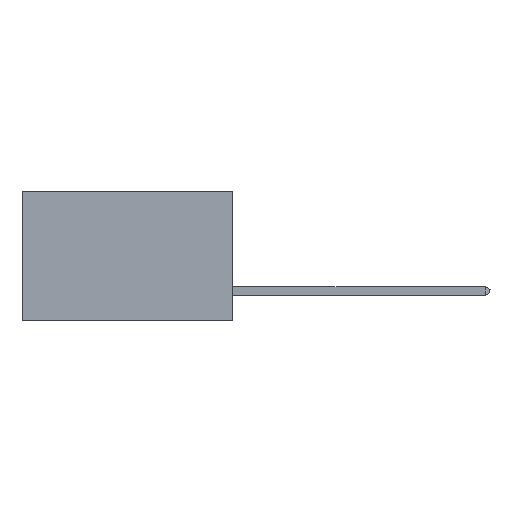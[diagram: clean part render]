
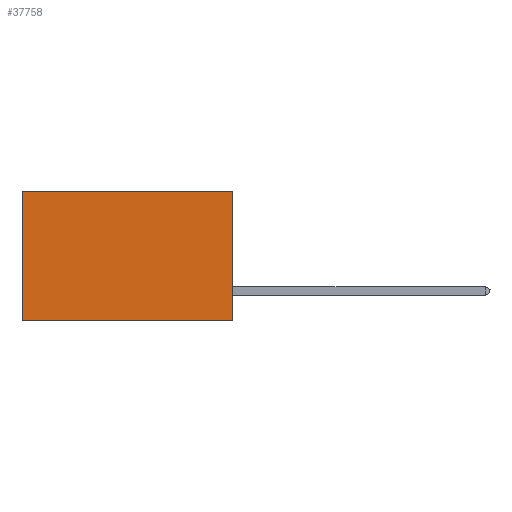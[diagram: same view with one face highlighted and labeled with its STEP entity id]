
A CAD part, left-side view. The second image highlights one B-rep face of the part: STEP entity #37758.
In plain terms, the highlighted planar face has unit normal (-1, 0, 0).
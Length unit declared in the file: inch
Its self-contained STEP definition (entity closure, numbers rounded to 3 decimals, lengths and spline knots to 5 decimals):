
#1246 = VERTEX_POINT ( 'NONE', #24276 ) ;
#2727 = CARTESIAN_POINT ( 'NONE',  ( 0.2875, 0., 0. ) ) ;
#3766 = PLANE ( 'NONE',  #4719 ) ;
#4719 = AXIS2_PLACEMENT_3D ( 'NONE', #18543, #32750, #11982 ) ;
#4760 = ORIENTED_EDGE ( 'NONE', *, *, #19969, .T. ) ;
#5701 = LINE ( 'NONE', #20849, #41844 ) ;
#6218 = DIRECTION ( 'NONE',  ( 0., 1., 0. ) ) ;
#7451 = VERTEX_POINT ( 'NONE', #17701 ) ;
#10800 = ORIENTED_EDGE ( 'NONE', *, *, #10847, .F. ) ;
#10847 = EDGE_CURVE ( 'NONE', #1246, #7451, #5701, .T. ) ;
#11982 = DIRECTION ( 'NONE',  ( 0., 0., -1. ) ) ;
#12939 = CARTESIAN_POINT ( 'NONE',  ( 0.2875, 0., 0. ) ) ;
#13552 = EDGE_LOOP ( 'NONE', ( #22248, #10800, #23681, #4760 ) ) ;
#15522 = CARTESIAN_POINT ( 'NONE',  ( 0.2875, 0.6, 0. ) ) ;
#17701 = CARTESIAN_POINT ( 'NONE',  ( 0.2875, 0.6, -0.37 ) ) ;
#18157 = VECTOR ( 'NONE', #29685, 39.37008 ) ;
#18256 = CARTESIAN_POINT ( 'NONE',  ( 0.2875, 0., 0. ) ) ;
#18543 = CARTESIAN_POINT ( 'NONE',  ( 0.2875, 0., 0. ) ) ;
#19969 = EDGE_CURVE ( 'NONE', #26157, #39459, #33981, .T. ) ;
#20849 = CARTESIAN_POINT ( 'NONE',  ( 0.2875, 0., -0.37 ) ) ;
#22248 = ORIENTED_EDGE ( 'NONE', *, *, #43045, .T. ) ;
#23681 = ORIENTED_EDGE ( 'NONE', *, *, #25748, .F. ) ;
#23796 = FACE_OUTER_BOUND ( 'NONE', #13552, .T. ) ;
#24276 = CARTESIAN_POINT ( 'NONE',  ( 0.2875, 0., -0.37 ) ) ;
#25748 = EDGE_CURVE ( 'NONE', #26157, #1246, #27617, .T. ) ;
#25964 = VECTOR ( 'NONE', #44663, 39.37008 ) ;
#26157 = VERTEX_POINT ( 'NONE', #12939 ) ;
#27617 = LINE ( 'NONE', #18256, #25964 ) ;
#29685 = DIRECTION ( 'NONE',  ( 0., 0., -1. ) ) ;
#32750 = DIRECTION ( 'NONE',  ( 1., 0., 0. ) ) ;
#33981 = LINE ( 'NONE', #2727, #34496 ) ;
#34496 = VECTOR ( 'NONE', #6218, 39.37008 ) ;
#36892 = LINE ( 'NONE', #15522, #18157 ) ;
#37758 = ADVANCED_FACE ( 'NONE', ( #23796 ), #3766, .F. ) ;
#38644 = DIRECTION ( 'NONE',  ( 0., 1., 0. ) ) ;
#39459 = VERTEX_POINT ( 'NONE', #44366 ) ;
#41844 = VECTOR ( 'NONE', #38644, 39.37008 ) ;
#43045 = EDGE_CURVE ( 'NONE', #39459, #7451, #36892, .T. ) ;
#44366 = CARTESIAN_POINT ( 'NONE',  ( 0.2875, 0.6, 0. ) ) ;
#44663 = DIRECTION ( 'NONE',  ( 0., 0., -1. ) ) ;
